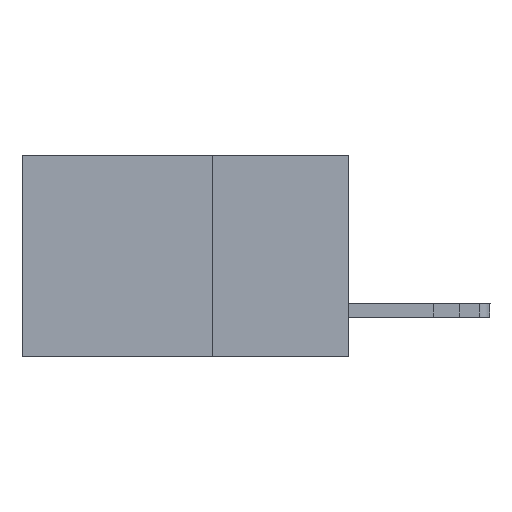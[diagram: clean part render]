
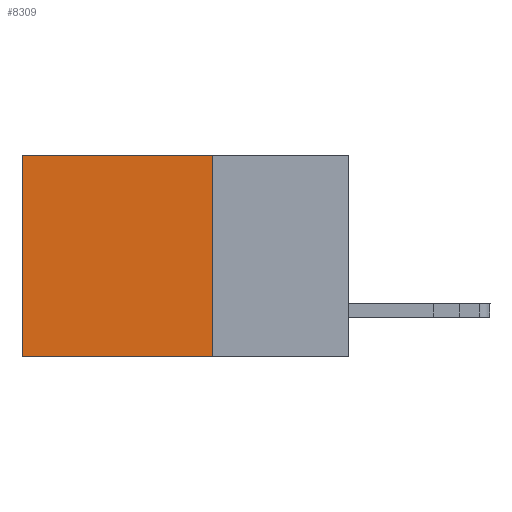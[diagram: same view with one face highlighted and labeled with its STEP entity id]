
A CAD part, left-side view. The second image highlights one B-rep face of the part: STEP entity #8309.
In plain terms, the highlighted planar face has unit normal (-1, 0, 0).
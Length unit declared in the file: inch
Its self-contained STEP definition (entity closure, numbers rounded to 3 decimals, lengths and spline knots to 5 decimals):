
#234 = CARTESIAN_POINT ( 'NONE',  ( 0.298, 0.6, 0. ) ) ;
#288 = FACE_OUTER_BOUND ( 'NONE', #10912, .T. ) ;
#967 = CARTESIAN_POINT ( 'NONE',  ( 0.298, 0.25, 0. ) ) ;
#1588 = AXIS2_PLACEMENT_3D ( 'NONE', #967, #12810, #10599 ) ;
#1690 = EDGE_CURVE ( 'NONE', #4143, #5717, #7768, .T. ) ;
#2066 = ORIENTED_EDGE ( 'NONE', *, *, #3163, .T. ) ;
#2243 = DIRECTION ( 'NONE',  ( 0., 0., -1. ) ) ;
#3163 = EDGE_CURVE ( 'NONE', #5717, #3802, #10231, .T. ) ;
#3458 = CARTESIAN_POINT ( 'NONE',  ( 0.298, 0.25, 0. ) ) ;
#3802 = VERTEX_POINT ( 'NONE', #8243 ) ;
#4143 = VERTEX_POINT ( 'NONE', #10676 ) ;
#5158 = ORIENTED_EDGE ( 'NONE', *, *, #1690, .T. ) ;
#5304 = EDGE_CURVE ( 'NONE', #4143, #7947, #6299, .T. ) ;
#5413 = DIRECTION ( 'NONE',  ( 0., 1., 0. ) ) ;
#5548 = LINE ( 'NONE', #12760, #7740 ) ;
#5717 = VERTEX_POINT ( 'NONE', #234 ) ;
#6299 = LINE ( 'NONE', #3458, #6459 ) ;
#6459 = VECTOR ( 'NONE', #13108, 39.37008 ) ;
#6762 = VECTOR ( 'NONE', #5413, 39.37008 ) ;
#6994 = CARTESIAN_POINT ( 'NONE',  ( 0.298, 0.25, -0.37 ) ) ;
#7463 = DIRECTION ( 'NONE',  ( 0., 1., 0. ) ) ;
#7740 = VECTOR ( 'NONE', #7463, 39.37008 ) ;
#7768 = LINE ( 'NONE', #11734, #6762 ) ;
#7947 = VERTEX_POINT ( 'NONE', #6994 ) ;
#8243 = CARTESIAN_POINT ( 'NONE',  ( 0.298, 0.6, -0.37 ) ) ;
#8309 = ADVANCED_FACE ( 'NONE', ( #288 ), #13896, .F. ) ;
#8715 = EDGE_CURVE ( 'NONE', #7947, #3802, #5548, .T. ) ;
#9050 = VECTOR ( 'NONE', #2243, 39.37008 ) ;
#10231 = LINE ( 'NONE', #12907, #9050 ) ;
#10599 = DIRECTION ( 'NONE',  ( 0., 0., -1. ) ) ;
#10676 = CARTESIAN_POINT ( 'NONE',  ( 0.298, 0.25, 0. ) ) ;
#10912 = EDGE_LOOP ( 'NONE', ( #2066, #10946, #13436, #5158 ) ) ;
#10946 = ORIENTED_EDGE ( 'NONE', *, *, #8715, .F. ) ;
#11734 = CARTESIAN_POINT ( 'NONE',  ( 0.298, 0.25, 0. ) ) ;
#12760 = CARTESIAN_POINT ( 'NONE',  ( 0.298, 0.25, -0.37 ) ) ;
#12810 = DIRECTION ( 'NONE',  ( 1., 0., 0. ) ) ;
#12907 = CARTESIAN_POINT ( 'NONE',  ( 0.298, 0.6, 0. ) ) ;
#13108 = DIRECTION ( 'NONE',  ( 0., 0., -1. ) ) ;
#13436 = ORIENTED_EDGE ( 'NONE', *, *, #5304, .F. ) ;
#13896 = PLANE ( 'NONE',  #1588 ) ;
